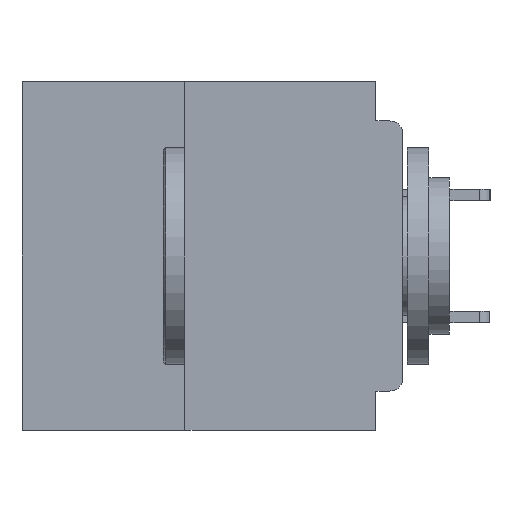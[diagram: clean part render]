
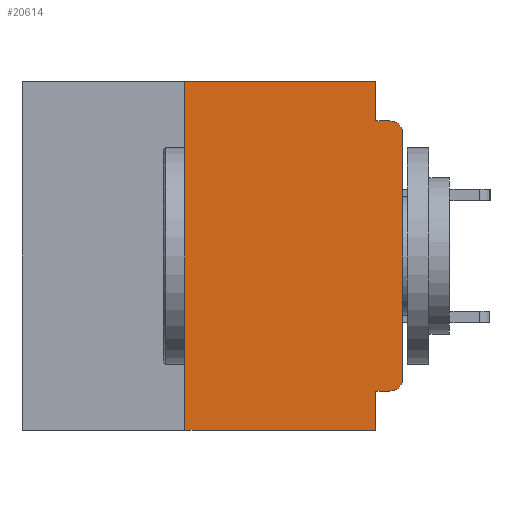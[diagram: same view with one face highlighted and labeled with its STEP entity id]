
A CAD part, left-side view. The second image highlights one B-rep face of the part: STEP entity #20614.
In plain terms, the highlighted planar face has unit normal (-1, 0, 0).
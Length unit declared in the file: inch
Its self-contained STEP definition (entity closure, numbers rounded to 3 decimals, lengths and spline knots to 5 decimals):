
#162 = AXIS2_PLACEMENT_3D ( 'NONE', #26586, #6495, #29929 ) ;
#308 = LINE ( 'NONE', #16492, #26040 ) ;
#665 = LINE ( 'NONE', #19576, #23233 ) ;
#1037 = CARTESIAN_POINT ( 'NONE',  ( 0., 0., -0.34 ) ) ;
#2375 = CARTESIAN_POINT ( 'NONE',  ( 0., 0.031, 0. ) ) ;
#2850 = DIRECTION ( 'NONE',  ( 0., 1., 0. ) ) ;
#3508 = LINE ( 'NONE', #39069, #10368 ) ;
#4038 = EDGE_CURVE ( 'NONE', #7260, #41854, #3508, .T. ) ;
#4206 = CARTESIAN_POINT ( 'NONE',  ( 0., 0.031, 0. ) ) ;
#5902 = DIRECTION ( 'NONE',  ( 0., 0., -1. ) ) ;
#6495 = DIRECTION ( 'NONE',  ( -1., 0., 0. ) ) ;
#7260 = VERTEX_POINT ( 'NONE', #7429 ) ;
#7429 = CARTESIAN_POINT ( 'NONE',  ( 0., 0.25, -0.4 ) ) ;
#7645 = FACE_OUTER_BOUND ( 'NONE', #16799, .T. ) ;
#7939 = CARTESIAN_POINT ( 'NONE',  ( 0., 0.015, -0.045 ) ) ;
#7955 = CARTESIAN_POINT ( 'NONE',  ( 0., 0., -0.06 ) ) ;
#8010 = DIRECTION ( 'NONE',  ( 0., -1., 0. ) ) ;
#8032 = ORIENTED_EDGE ( 'NONE', *, *, #10780, .F. ) ;
#9603 = LINE ( 'NONE', #2375, #35204 ) ;
#9734 = VECTOR ( 'NONE', #5902, 39.37008 ) ;
#10047 = CARTESIAN_POINT ( 'NONE',  ( 0., 0.015, -0.355 ) ) ;
#10241 = CARTESIAN_POINT ( 'NONE',  ( 0., 0.437, 0. ) ) ;
#10368 = VECTOR ( 'NONE', #38648, 39.37008 ) ;
#10535 = ORIENTED_EDGE ( 'NONE', *, *, #15924, .T. ) ;
#10780 = EDGE_CURVE ( 'NONE', #24567, #37283, #665, .T. ) ;
#11769 = VERTEX_POINT ( 'NONE', #7939 ) ;
#12848 = VECTOR ( 'NONE', #24044, 39.37008 ) ;
#13410 = EDGE_CURVE ( 'NONE', #40054, #17318, #24620, .T. ) ;
#13445 = ORIENTED_EDGE ( 'NONE', *, *, #40646, .T. ) ;
#13627 = DIRECTION ( 'NONE',  ( 0., 0., -1. ) ) ;
#14161 = ORIENTED_EDGE ( 'NONE', *, *, #16724, .F. ) ;
#15522 = ORIENTED_EDGE ( 'NONE', *, *, #4038, .F. ) ;
#15924 = EDGE_CURVE ( 'NONE', #7260, #28697, #39376, .T. ) ;
#16410 = DIRECTION ( 'NONE',  ( 0., 0., 1. ) ) ;
#16492 = CARTESIAN_POINT ( 'NONE',  ( 0., 0., -0.045 ) ) ;
#16724 = EDGE_CURVE ( 'NONE', #41854, #35011, #17982, .T. ) ;
#16799 = EDGE_LOOP ( 'NONE', ( #28011, #13445, #27188, #30366, #14161, #15522, #10535, #39896, #8032, #27276 ) ) ;
#16918 = EDGE_CURVE ( 'NONE', #35011, #30314, #9603, .T. ) ;
#17169 = DIRECTION ( 'NONE',  ( -1., 0., 0. ) ) ;
#17318 = VERTEX_POINT ( 'NONE', #7955 ) ;
#17799 = AXIS2_PLACEMENT_3D ( 'NONE', #10241, #33609, #13627 ) ;
#17982 = LINE ( 'NONE', #28077, #34696 ) ;
#18618 = LINE ( 'NONE', #35862, #9734 ) ;
#19576 = CARTESIAN_POINT ( 'NONE',  ( 0., 0., -0.355 ) ) ;
#20614 = ADVANCED_FACE ( 'NONE', ( #7645 ), #23556, .F. ) ;
#21000 = EDGE_CURVE ( 'NONE', #37283, #28697, #18618, .T. ) ;
#22987 = CARTESIAN_POINT ( 'NONE',  ( 0., 0., 0. ) ) ;
#23233 = VECTOR ( 'NONE', #2850, 39.37008 ) ;
#23556 = PLANE ( 'NONE',  #17799 ) ;
#23582 = VECTOR ( 'NONE', #16410, 39.37008 ) ;
#24044 = DIRECTION ( 'NONE',  ( 0., -1., 0. ) ) ;
#24458 = CIRCLE ( 'NONE', #26930, 0.015 ) ;
#24536 = EDGE_CURVE ( 'NONE', #24567, #40054, #42851, .T. ) ;
#24567 = VERTEX_POINT ( 'NONE', #10047 ) ;
#24620 = LINE ( 'NONE', #22987, #23582 ) ;
#26040 = VECTOR ( 'NONE', #39761, 39.37008 ) ;
#26586 = CARTESIAN_POINT ( 'NONE',  ( 0., 0.015, -0.34 ) ) ;
#26930 = AXIS2_PLACEMENT_3D ( 'NONE', #37127, #17169, #40449 ) ;
#27188 = ORIENTED_EDGE ( 'NONE', *, *, #31332, .F. ) ;
#27276 = ORIENTED_EDGE ( 'NONE', *, *, #24536, .T. ) ;
#27708 = CARTESIAN_POINT ( 'NONE',  ( 0., 0.031, -0.045 ) ) ;
#28011 = ORIENTED_EDGE ( 'NONE', *, *, #13410, .T. ) ;
#28077 = CARTESIAN_POINT ( 'NONE',  ( 0., 0.437, 0. ) ) ;
#28697 = VERTEX_POINT ( 'NONE', #32639 ) ;
#28841 = CARTESIAN_POINT ( 'NONE',  ( 0., 0.031, -0.355 ) ) ;
#29269 = CARTESIAN_POINT ( 'NONE',  ( 0., 0.25, 0. ) ) ;
#29929 = DIRECTION ( 'NONE',  ( 0., 0., -1. ) ) ;
#30314 = VERTEX_POINT ( 'NONE', #27708 ) ;
#30366 = ORIENTED_EDGE ( 'NONE', *, *, #16918, .F. ) ;
#31332 = EDGE_CURVE ( 'NONE', #30314, #11769, #308, .T. ) ;
#32639 = CARTESIAN_POINT ( 'NONE',  ( 0., 0.031, -0.4 ) ) ;
#33609 = DIRECTION ( 'NONE',  ( 1., 0., 0. ) ) ;
#34696 = VECTOR ( 'NONE', #8010, 39.37008 ) ;
#35011 = VERTEX_POINT ( 'NONE', #4206 ) ;
#35204 = VECTOR ( 'NONE', #42381, 39.37008 ) ;
#35862 = CARTESIAN_POINT ( 'NONE',  ( 0., 0.031, -0.4 ) ) ;
#37127 = CARTESIAN_POINT ( 'NONE',  ( 0., 0.015, -0.06 ) ) ;
#37283 = VERTEX_POINT ( 'NONE', #28841 ) ;
#37403 = CARTESIAN_POINT ( 'NONE',  ( 0., 0.437, -0.4 ) ) ;
#38648 = DIRECTION ( 'NONE',  ( 0., 0., 1. ) ) ;
#39069 = CARTESIAN_POINT ( 'NONE',  ( 0., 0.25, -0.4 ) ) ;
#39376 = LINE ( 'NONE', #37403, #12848 ) ;
#39761 = DIRECTION ( 'NONE',  ( 0., -1., 0. ) ) ;
#39896 = ORIENTED_EDGE ( 'NONE', *, *, #21000, .F. ) ;
#40054 = VERTEX_POINT ( 'NONE', #1037 ) ;
#40449 = DIRECTION ( 'NONE',  ( 0., 0., -1. ) ) ;
#40646 = EDGE_CURVE ( 'NONE', #17318, #11769, #24458, .T. ) ;
#41854 = VERTEX_POINT ( 'NONE', #29269 ) ;
#42381 = DIRECTION ( 'NONE',  ( 0., 0., -1. ) ) ;
#42851 = CIRCLE ( 'NONE', #162, 0.015 ) ;
